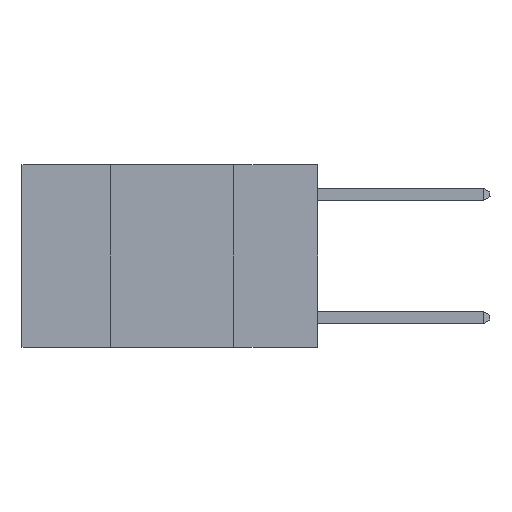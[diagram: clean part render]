
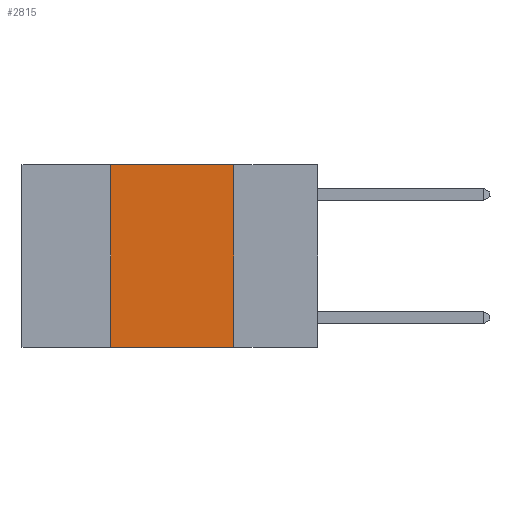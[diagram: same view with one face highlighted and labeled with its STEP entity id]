
A CAD part, left-side view. The second image highlights one B-rep face of the part: STEP entity #2815.
In plain terms, the highlighted planar face has unit normal (-1, 0, 0).
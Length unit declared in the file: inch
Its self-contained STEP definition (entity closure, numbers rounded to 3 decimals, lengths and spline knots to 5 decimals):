
#2 = ORIENTED_EDGE ( 'NONE', *, *, #8215, .F. ) ;
#81 = VERTEX_POINT ( 'NONE', #6353 ) ;
#148 = CARTESIAN_POINT ( 'NONE',  ( 0., 0.42, -0.37 ) ) ;
#387 = FACE_OUTER_BOUND ( 'NONE', #6070, .T. ) ;
#388 = LINE ( 'NONE', #6917, #4342 ) ;
#561 = DIRECTION ( 'NONE',  ( 0., 0., -1. ) ) ;
#906 = ORIENTED_EDGE ( 'NONE', *, *, #8155, .F. ) ;
#1506 = DIRECTION ( 'NONE',  ( 0., -1., 0. ) ) ;
#2392 = CARTESIAN_POINT ( 'NONE',  ( 0., 0.17, -0.37 ) ) ;
#2536 = CARTESIAN_POINT ( 'NONE',  ( 0., 0.6, 0. ) ) ;
#2815 = ADVANCED_FACE ( 'NONE', ( #387 ), #8204, .F. ) ;
#2899 = VECTOR ( 'NONE', #6787, 39.37008 ) ;
#3324 = DIRECTION ( 'NONE',  ( 1., 0., 0. ) ) ;
#3867 = LINE ( 'NONE', #8714, #10120 ) ;
#4342 = VECTOR ( 'NONE', #561, 39.37008 ) ;
#4375 = ORIENTED_EDGE ( 'NONE', *, *, #7651, .F. ) ;
#4562 = VERTEX_POINT ( 'NONE', #8972 ) ;
#4577 = CARTESIAN_POINT ( 'NONE',  ( 0., 0.42, 0. ) ) ;
#5159 = CARTESIAN_POINT ( 'NONE',  ( 0., 0.6, 0. ) ) ;
#5390 = DIRECTION ( 'NONE',  ( 0., 0., 1. ) ) ;
#5917 = ORIENTED_EDGE ( 'NONE', *, *, #8218, .T. ) ;
#6070 = EDGE_LOOP ( 'NONE', ( #906, #4375, #2, #5917 ) ) ;
#6353 = CARTESIAN_POINT ( 'NONE',  ( 0., 0.17, 0. ) ) ;
#6787 = DIRECTION ( 'NONE',  ( 0., -1., 0. ) ) ;
#6917 = CARTESIAN_POINT ( 'NONE',  ( 0., 0.17, 0. ) ) ;
#7651 = EDGE_CURVE ( 'NONE', #4562, #81, #9365, .T. ) ;
#7875 = AXIS2_PLACEMENT_3D ( 'NONE', #2536, #3324, #9000 ) ;
#8155 = EDGE_CURVE ( 'NONE', #81, #9283, #388, .T. ) ;
#8204 = PLANE ( 'NONE',  #7875 ) ;
#8215 = EDGE_CURVE ( 'NONE', #10316, #4562, #8493, .T. ) ;
#8218 = EDGE_CURVE ( 'NONE', #10316, #9283, #3867, .T. ) ;
#8231 = VECTOR ( 'NONE', #5390, 39.37008 ) ;
#8493 = LINE ( 'NONE', #4577, #8231 ) ;
#8714 = CARTESIAN_POINT ( 'NONE',  ( 0., 0.6, -0.37 ) ) ;
#8972 = CARTESIAN_POINT ( 'NONE',  ( 0., 0.42, 0. ) ) ;
#9000 = DIRECTION ( 'NONE',  ( 0., 0., -1. ) ) ;
#9283 = VERTEX_POINT ( 'NONE', #2392 ) ;
#9365 = LINE ( 'NONE', #5159, #2899 ) ;
#10120 = VECTOR ( 'NONE', #1506, 39.37008 ) ;
#10316 = VERTEX_POINT ( 'NONE', #148 ) ;
